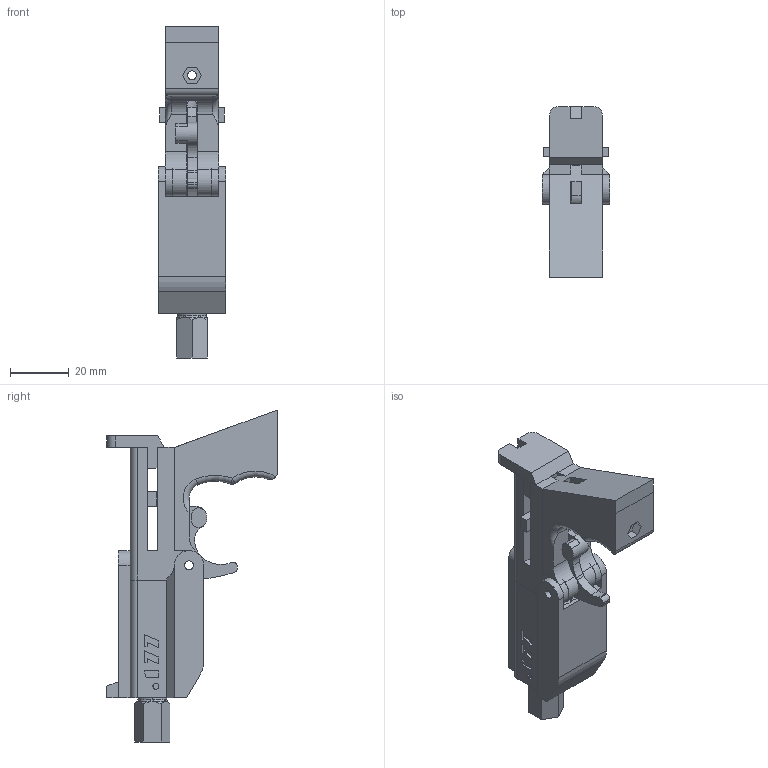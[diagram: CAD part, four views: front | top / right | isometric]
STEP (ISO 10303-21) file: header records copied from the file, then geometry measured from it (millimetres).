
FILE_DESCRIPTION (( 'STEP AP214' ), '1' );
FILE_NAME ('CabooseParlor.STEP', '2014-10-07T00:00:22', ( 'WarFairy' ), ( '' ), 'SwSTEP 2.0', 'SolidWorks 2013', '' );
FILE_SCHEMA (( 'AUTOMOTIVE_DESIGN' ));
Length unit declared in the file: millimetre
Products named in the file (8): RearPlateS^CabooseParlor; Barrel111^Launcher; ParlorMod^CabooseParlor; TriggerModF^CabooseParlor; Grip^Launcher2; Bolt^CabooseParlor; Body; CabooseParlor
Assembly tree (7 placements, depth 2):
  CabooseParlor
    Body
    Bolt^CabooseParlor
    Grip^Launcher2
    TriggerModF^CabooseParlor
    ParlorMod^CabooseParlor
    Barrel111^Launcher
    RearPlateS^CabooseParlor
Bounding box: 23 x 58 x 112.73 mm (x, y, z)
Volume: 46543.3 mm3; surface area: 23791.1 mm2
Topology: 7 solids, 7 shells, 474 faces, 1275 edges, 838 vertices
Faces by surface type: plane 286, cylinder 94, bspline 74, torus 12, cone 8
Entity records: 18486 total; most frequent: CARTESIAN_POINT 6588, ORIENTED_EDGE 2546, DIRECTION 2137, EDGE_CURVE 1273, VECTOR 875, LINE 875, VERTEX_POINT 838, AXIS2_PLACEMENT_3D 631
